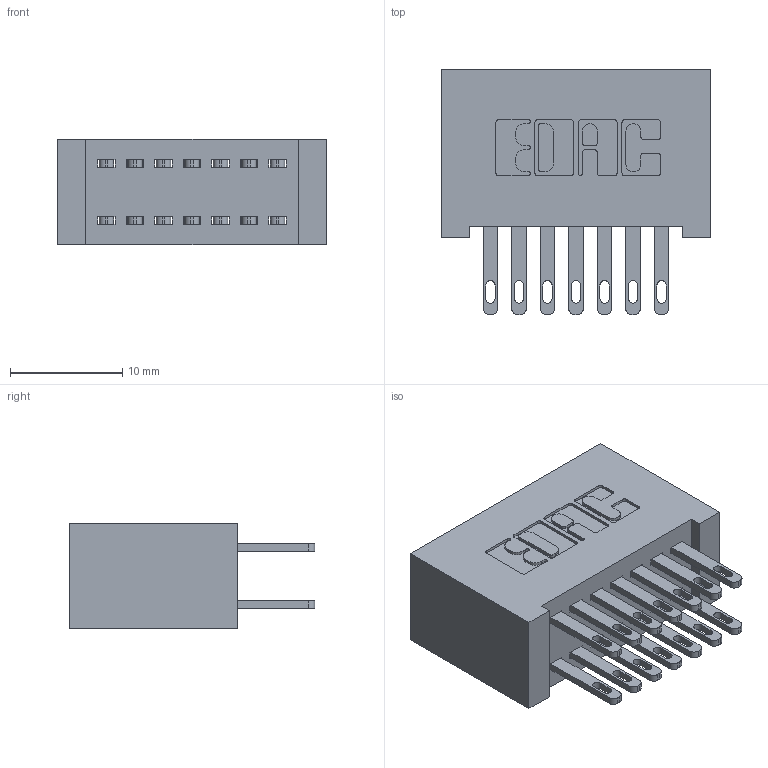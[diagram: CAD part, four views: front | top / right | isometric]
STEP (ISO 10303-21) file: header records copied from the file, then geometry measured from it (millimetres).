
FILE_DESCRIPTION (( 'STEP AP203' ), '1' );
FILE_NAME ('342-014-500-201.STEP', '2019-10-01T16:18:13', ( '' ), ( '' ), 'SwSTEP 2.0', 'SolidWorks 2016', '' );
FILE_SCHEMA (( 'CONFIG_CONTROL_DESIGN' ));
Length unit declared in the file: inch
Products named in the file (3): 342 Part_Lugless; 345-292-001_345-293-100; 342-014-500-201
Assembly tree (15 placements, depth 2):
  342-014-500-201
    342 Part_Lugless
    345-292-001_345-293-100  x14
Bounding box: 24.03 x 21.85 x 9.4 mm (x, y, z)
Volume: 2475.6 mm3; surface area: 3747.5 mm2
Topology: 15 solids, 15 shells, 774 faces, 2333 edges, 1554 vertices
Faces by surface type: plane 482, cylinder 292
Entity records: 8551 total; most frequent: CARTESIAN_POINT 1454, ORIENTED_EDGE 1390, DIRECTION 1299, EDGE_CURVE 695, LINE 571, VECTOR 571, VERTEX_POINT 462, AXIS2_PLACEMENT_3D 364
